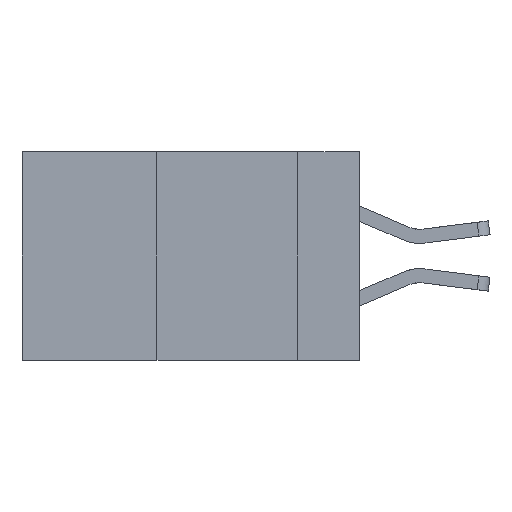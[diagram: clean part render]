
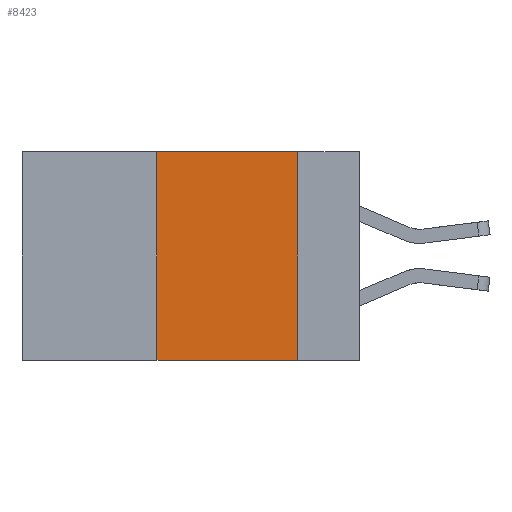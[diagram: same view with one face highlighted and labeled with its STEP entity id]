
A CAD part, left-side view. The second image highlights one B-rep face of the part: STEP entity #8423.
In plain terms, the highlighted planar face has unit normal (-1, 0, 0).
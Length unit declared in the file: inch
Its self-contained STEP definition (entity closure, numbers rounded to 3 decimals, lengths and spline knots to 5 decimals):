
#124 = DIRECTION ( 'NONE',  ( 0., -1., 0. ) ) ;
#146 = EDGE_CURVE ( 'NONE', #7226, #6930, #7460, .T. ) ;
#320 = VERTEX_POINT ( 'NONE', #1224 ) ;
#965 = CARTESIAN_POINT ( 'NONE',  ( 0., 0.36, 0. ) ) ;
#1224 = CARTESIAN_POINT ( 'NONE',  ( 0., 0.36, -0.37 ) ) ;
#1336 = DIRECTION ( 'NONE',  ( 0., 0., 1. ) ) ;
#1684 = DIRECTION ( 'NONE',  ( 0., 0., -1. ) ) ;
#2249 = EDGE_CURVE ( 'NONE', #320, #5720, #2810, .T. ) ;
#2261 = ORIENTED_EDGE ( 'NONE', *, *, #8142, .F. ) ;
#2810 = LINE ( 'NONE', #4455, #6499 ) ;
#2815 = CARTESIAN_POINT ( 'NONE',  ( 0., 0.11, 0. ) ) ;
#3140 = DIRECTION ( 'NONE',  ( 1., 0., 0. ) ) ;
#3556 = DIRECTION ( 'NONE',  ( 0., -1., 0. ) ) ;
#3757 = VECTOR ( 'NONE', #1336, 39.37008 ) ;
#4185 = LINE ( 'NONE', #7232, #6644 ) ;
#4311 = LINE ( 'NONE', #9992, #3757 ) ;
#4455 = CARTESIAN_POINT ( 'NONE',  ( 0., 0.6, -0.37 ) ) ;
#4573 = PLANE ( 'NONE',  #7123 ) ;
#4781 = FACE_OUTER_BOUND ( 'NONE', #7291, .T. ) ;
#5630 = DIRECTION ( 'NONE',  ( 0., 0., -1. ) ) ;
#5720 = VERTEX_POINT ( 'NONE', #7242 ) ;
#6499 = VECTOR ( 'NONE', #3556, 39.37008 ) ;
#6627 = CARTESIAN_POINT ( 'NONE',  ( 0., 0.6, 0. ) ) ;
#6644 = VECTOR ( 'NONE', #1684, 39.37008 ) ;
#6832 = ORIENTED_EDGE ( 'NONE', *, *, #9892, .F. ) ;
#6930 = VERTEX_POINT ( 'NONE', #2815 ) ;
#7123 = AXIS2_PLACEMENT_3D ( 'NONE', #7781, #3140, #5630 ) ;
#7226 = VERTEX_POINT ( 'NONE', #965 ) ;
#7232 = CARTESIAN_POINT ( 'NONE',  ( 0., 0.11, 0. ) ) ;
#7242 = CARTESIAN_POINT ( 'NONE',  ( 0., 0.11, -0.37 ) ) ;
#7291 = EDGE_LOOP ( 'NONE', ( #6832, #9134, #2261, #8174 ) ) ;
#7460 = LINE ( 'NONE', #6627, #10051 ) ;
#7781 = CARTESIAN_POINT ( 'NONE',  ( 0., 0.6, 0. ) ) ;
#8142 = EDGE_CURVE ( 'NONE', #320, #7226, #4311, .T. ) ;
#8174 = ORIENTED_EDGE ( 'NONE', *, *, #2249, .T. ) ;
#8423 = ADVANCED_FACE ( 'NONE', ( #4781 ), #4573, .F. ) ;
#9134 = ORIENTED_EDGE ( 'NONE', *, *, #146, .F. ) ;
#9892 = EDGE_CURVE ( 'NONE', #6930, #5720, #4185, .T. ) ;
#9992 = CARTESIAN_POINT ( 'NONE',  ( 0., 0.36, 0. ) ) ;
#10051 = VECTOR ( 'NONE', #124, 39.37008 ) ;
